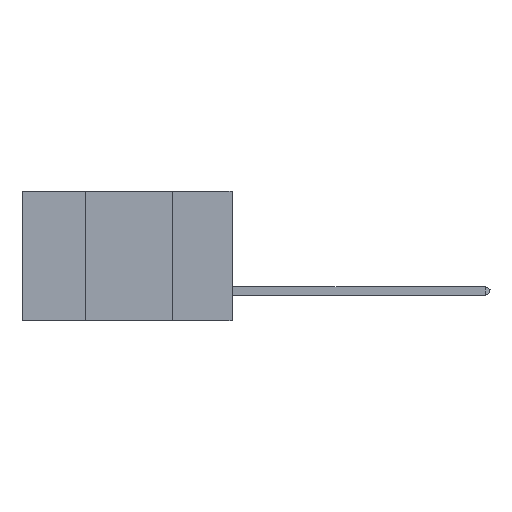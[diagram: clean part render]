
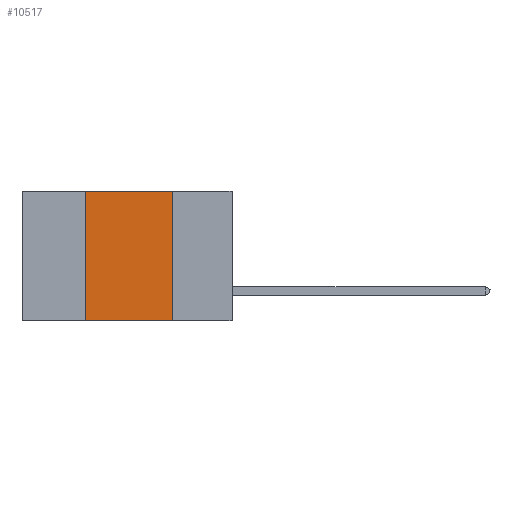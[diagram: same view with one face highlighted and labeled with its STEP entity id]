
A CAD part, left-side view. The second image highlights one B-rep face of the part: STEP entity #10517.
In plain terms, the highlighted planar face has unit normal (-1, 0, 0).
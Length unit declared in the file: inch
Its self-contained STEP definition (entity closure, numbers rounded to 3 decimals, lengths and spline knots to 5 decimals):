
#1264 = LINE ( 'NONE', #18012, #11561 ) ;
#2189 = EDGE_CURVE ( 'NONE', #19750, #27860, #28235, .T. ) ;
#2720 = EDGE_CURVE ( 'NONE', #27860, #17317, #7899, .T. ) ;
#3218 = DIRECTION ( 'NONE',  ( 0., 0., 1. ) ) ;
#3404 = ORIENTED_EDGE ( 'NONE', *, *, #2189, .F. ) ;
#4165 = ORIENTED_EDGE ( 'NONE', *, *, #9163, .F. ) ;
#4885 = VECTOR ( 'NONE', #22134, 39.37008 ) ;
#5346 = EDGE_CURVE ( 'NONE', #19750, #19470, #1264, .T. ) ;
#6165 = LINE ( 'NONE', #11113, #4885 ) ;
#7785 = CARTESIAN_POINT ( 'NONE',  ( 0., 0.42, -0.37 ) ) ;
#7899 = LINE ( 'NONE', #11530, #29527 ) ;
#9163 = EDGE_CURVE ( 'NONE', #17317, #19470, #6165, .T. ) ;
#9762 = ORIENTED_EDGE ( 'NONE', *, *, #2720, .F. ) ;
#10517 = ADVANCED_FACE ( 'NONE', ( #18148 ), #25864, .F. ) ;
#11113 = CARTESIAN_POINT ( 'NONE',  ( 0., 0.17, 0. ) ) ;
#11530 = CARTESIAN_POINT ( 'NONE',  ( 0., 0.6, 0. ) ) ;
#11561 = VECTOR ( 'NONE', #20535, 39.37008 ) ;
#13946 = CARTESIAN_POINT ( 'NONE',  ( 0., 0.42, 0. ) ) ;
#17317 = VERTEX_POINT ( 'NONE', #31406 ) ;
#17700 = DIRECTION ( 'NONE',  ( 0., 0., -1. ) ) ;
#18012 = CARTESIAN_POINT ( 'NONE',  ( 0., 0.6, -0.37 ) ) ;
#18148 = FACE_OUTER_BOUND ( 'NONE', #19438, .T. ) ;
#19438 = EDGE_LOOP ( 'NONE', ( #4165, #9762, #3404, #35788 ) ) ;
#19470 = VERTEX_POINT ( 'NONE', #23190 ) ;
#19750 = VERTEX_POINT ( 'NONE', #7785 ) ;
#20535 = DIRECTION ( 'NONE',  ( 0., -1., 0. ) ) ;
#21399 = AXIS2_PLACEMENT_3D ( 'NONE', #31429, #34353, #17700 ) ;
#22134 = DIRECTION ( 'NONE',  ( 0., 0., -1. ) ) ;
#22422 = DIRECTION ( 'NONE',  ( 0., -1., 0. ) ) ;
#23190 = CARTESIAN_POINT ( 'NONE',  ( 0., 0.17, -0.37 ) ) ;
#25864 = PLANE ( 'NONE',  #21399 ) ;
#27860 = VERTEX_POINT ( 'NONE', #33545 ) ;
#28235 = LINE ( 'NONE', #13946, #31224 ) ;
#29527 = VECTOR ( 'NONE', #22422, 39.37008 ) ;
#31224 = VECTOR ( 'NONE', #3218, 39.37008 ) ;
#31406 = CARTESIAN_POINT ( 'NONE',  ( 0., 0.17, 0. ) ) ;
#31429 = CARTESIAN_POINT ( 'NONE',  ( 0., 0.6, 0. ) ) ;
#33545 = CARTESIAN_POINT ( 'NONE',  ( 0., 0.42, 0. ) ) ;
#34353 = DIRECTION ( 'NONE',  ( 1., 0., 0. ) ) ;
#35788 = ORIENTED_EDGE ( 'NONE', *, *, #5346, .T. ) ;
